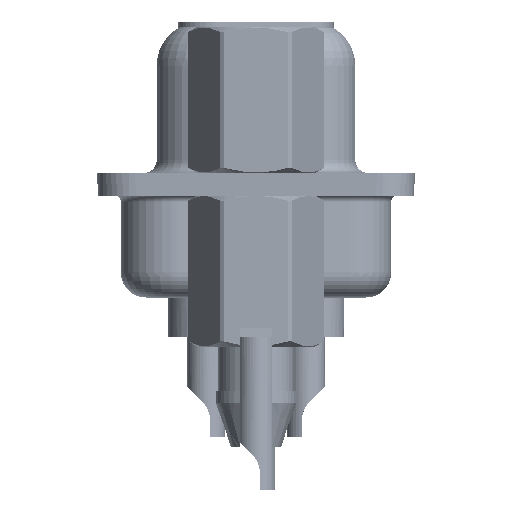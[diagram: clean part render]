
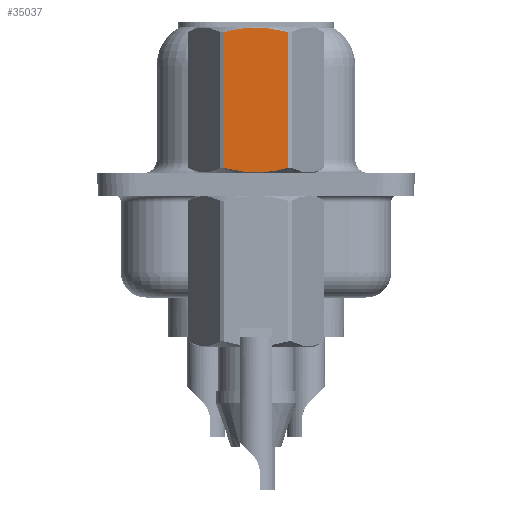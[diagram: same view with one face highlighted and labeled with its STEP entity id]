
A CAD part, left-side view. The second image highlights one B-rep face of the part: STEP entity #35037.
In plain terms, the highlighted planar face has unit normal (-1, 0, 0).
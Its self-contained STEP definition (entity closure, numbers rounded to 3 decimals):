
#890 = ORIENTED_EDGE ( 'NONE', *, *, #23447, .T. ) ;
#2666 = CARTESIAN_POINT ( 'NONE',  ( -2.381, 1.273, 6.048 ) ) ;
#2909 = CARTESIAN_POINT ( 'NONE',  ( -2.381, -0.215, 6.232 ) ) ;
#5336 = CARTESIAN_POINT ( 'NONE',  ( -2.381, -1.066, 0.596 ) ) ;
#6184 = VERTEX_POINT ( 'NONE', #46144 ) ;
#6418 = CARTESIAN_POINT ( 'NONE',  ( -2.381, 0.215, 6.232 ) ) ;
#6541 = PLANE ( 'NONE',  #46651 ) ;
#6663 = CARTESIAN_POINT ( 'NONE',  ( -2.381, -0.432, 6.215 ) ) ;
#6913 = CARTESIAN_POINT ( 'NONE',  ( -2.381, 1.065, 6.104 ) ) ;
#7029 = DIRECTION ( 'NONE',  ( 0., -1., 0. ) ) ;
#7290 = VERTEX_POINT ( 'NONE', #46297 ) ;
#8830 = CARTESIAN_POINT ( 'NONE',  ( -2.381, 1.065, 0.596 ) ) ;
#9063 = CARTESIAN_POINT ( 'NONE',  ( -2.381, -0.215, 0.468 ) ) ;
#9606 = EDGE_CURVE ( 'NONE', #6184, #7290, #40566, .T. ) ;
#10027 = CARTESIAN_POINT ( 'NONE',  ( -2.381, 1.375, -3.75 ) ) ;
#14846 = CARTESIAN_POINT ( 'NONE',  ( -2.381, 1.273, 6.048 ) ) ;
#17058 = LINE ( 'NONE', #32202, #47716 ) ;
#19223 = EDGE_CURVE ( 'NONE', #7290, #30835, #17058, .T. ) ;
#20240 = CARTESIAN_POINT ( 'NONE',  ( -2.381, 1.273, 0.652 ) ) ;
#20903 = VERTEX_POINT ( 'NONE', #14846 ) ;
#21076 = CARTESIAN_POINT ( 'NONE',  ( -2.381, -1.066, 6.104 ) ) ;
#21687 = DIRECTION ( 'NONE',  ( -1., 0., 0. ) ) ;
#23447 = EDGE_CURVE ( 'NONE', #20903, #6184, #37559, .T. ) ;
#23998 = CARTESIAN_POINT ( 'NONE',  ( -2.381, 0.215, 0.468 ) ) ;
#24980 = CARTESIAN_POINT ( 'NONE',  ( -2.381, 0.428, 0.485 ) ) ;
#25925 = FACE_OUTER_BOUND ( 'NONE', #37048, .T. ) ;
#27806 = ORIENTED_EDGE ( 'NONE', *, *, #19223, .T. ) ;
#28536 = CARTESIAN_POINT ( 'NONE',  ( -2.381, -0.858, 6.15 ) ) ;
#28691 = CARTESIAN_POINT ( 'NONE',  ( -2.381, 0.853, 0.549 ) ) ;
#29016 = CARTESIAN_POINT ( 'NONE',  ( -2.381, 0.853, 6.151 ) ) ;
#30835 = VERTEX_POINT ( 'NONE', #41511 ) ;
#32202 = CARTESIAN_POINT ( 'NONE',  ( -2.381, -1.273, 3.792 ) ) ;
#32270 = ORIENTED_EDGE ( 'NONE', *, *, #9606, .T. ) ;
#35037 = ADVANCED_FACE ( 'NONE', ( #25925 ), #6541, .T. ) ;
#35707 = CARTESIAN_POINT ( 'NONE',  ( -2.381, -1.273, 0.652 ) ) ;
#35858 = EDGE_CURVE ( 'NONE', #30835, #20903, #43138, .T. ) ;
#36781 = CARTESIAN_POINT ( 'NONE',  ( -2.381, 0.428, 6.215 ) ) ;
#37048 = EDGE_LOOP ( 'NONE', ( #32270, #27806, #45992, #890 ) ) ;
#37559 = LINE ( 'NONE', #48535, #43659 ) ;
#39195 = CARTESIAN_POINT ( 'NONE',  ( -2.381, -0.432, 0.485 ) ) ;
#39448 = CARTESIAN_POINT ( 'NONE',  ( -2.381, -0.858, 0.55 ) ) ;
#40566 = B_SPLINE_CURVE_WITH_KNOTS ( 'NONE', 3,
 ( #20240, #8830, #28691, #24980, #23998, #9063, #39195, #39448, #5336, #35707 ),
 .UNSPECIFIED., .F., .F.,
 ( 4, 2, 2, 2, 4 ),
 ( 0.003, 0.003, 0.004, 0.004, 0.005 ),
 .UNSPECIFIED. ) ;
#40589 = DIRECTION ( 'NONE',  ( 0., 0., -1. ) ) ;
#41511 = CARTESIAN_POINT ( 'NONE',  ( -2.381, -1.273, 6.048 ) ) ;
#43138 = B_SPLINE_CURVE_WITH_KNOTS ( 'NONE', 3,
 ( #44004, #21076, #28536, #6663, #2909, #6418, #36781, #29016, #6913, #2666 ),
 .UNSPECIFIED., .F., .F.,
 ( 4, 2, 2, 2, 4 ),
 ( 0.001, 0.002, 0.002, 0.003, 0.004 ),
 .UNSPECIFIED. ) ;
#43659 = VECTOR ( 'NONE', #40589, 1000. ) ;
#44004 = CARTESIAN_POINT ( 'NONE',  ( -2.381, -1.273, 6.048 ) ) ;
#45992 = ORIENTED_EDGE ( 'NONE', *, *, #35858, .T. ) ;
#46144 = CARTESIAN_POINT ( 'NONE',  ( -2.381, 1.273, 0.652 ) ) ;
#46297 = CARTESIAN_POINT ( 'NONE',  ( -2.381, -1.273, 0.652 ) ) ;
#46651 = AXIS2_PLACEMENT_3D ( 'NONE', #10027, #21687, #7029 ) ;
#47444 = DIRECTION ( 'NONE',  ( 0., 0., 1. ) ) ;
#47716 = VECTOR ( 'NONE', #47444, 1000. ) ;
#48535 = CARTESIAN_POINT ( 'NONE',  ( -2.381, 1.273, 3.792 ) ) ;
